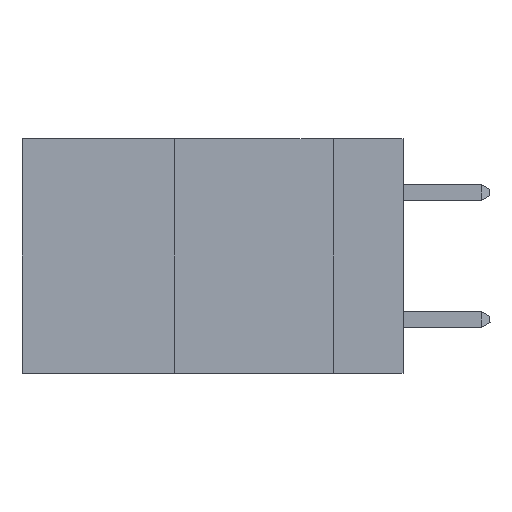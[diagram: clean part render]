
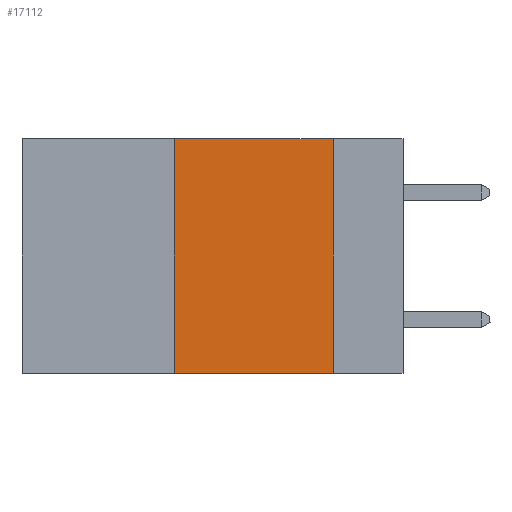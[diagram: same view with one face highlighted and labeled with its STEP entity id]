
A CAD part, left-side view. The second image highlights one B-rep face of the part: STEP entity #17112.
In plain terms, the highlighted planar face has unit normal (-1, 0, 0).
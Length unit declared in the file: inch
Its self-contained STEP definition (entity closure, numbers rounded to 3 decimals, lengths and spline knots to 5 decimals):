
#1126 = VERTEX_POINT ( 'NONE', #2800 ) ;
#1884 = CARTESIAN_POINT ( 'NONE',  ( 0., 0.11, -0.37 ) ) ;
#2019 = EDGE_CURVE ( 'NONE', #4057, #1126, #20862, .T. ) ;
#2583 = PLANE ( 'NONE',  #6562 ) ;
#2800 = CARTESIAN_POINT ( 'NONE',  ( 0., 0.36, 0. ) ) ;
#3317 = CARTESIAN_POINT ( 'NONE',  ( 0., 0.11, 0. ) ) ;
#3446 = EDGE_CURVE ( 'NONE', #4057, #5970, #21675, .T. ) ;
#4057 = VERTEX_POINT ( 'NONE', #12429 ) ;
#5388 = CARTESIAN_POINT ( 'NONE',  ( 0., 0.6, 0. ) ) ;
#5970 = VERTEX_POINT ( 'NONE', #1884 ) ;
#6185 = DIRECTION ( 'NONE',  ( 0., 0., -1. ) ) ;
#6562 = AXIS2_PLACEMENT_3D ( 'NONE', #5388, #20979, #11325 ) ;
#6912 = VERTEX_POINT ( 'NONE', #3317 ) ;
#6990 = VECTOR ( 'NONE', #25019, 39.37008 ) ;
#7381 = ORIENTED_EDGE ( 'NONE', *, *, #16291, .F. ) ;
#7469 = ORIENTED_EDGE ( 'NONE', *, *, #2019, .F. ) ;
#7756 = ORIENTED_EDGE ( 'NONE', *, *, #3446, .T. ) ;
#8862 = VECTOR ( 'NONE', #11397, 39.37008 ) ;
#9493 = DIRECTION ( 'NONE',  ( 0., 0., 1. ) ) ;
#11325 = DIRECTION ( 'NONE',  ( 0., 0., -1. ) ) ;
#11397 = DIRECTION ( 'NONE',  ( 0., -1., 0. ) ) ;
#11401 = ORIENTED_EDGE ( 'NONE', *, *, #12541, .F. ) ;
#12429 = CARTESIAN_POINT ( 'NONE',  ( 0., 0.36, -0.37 ) ) ;
#12541 = EDGE_CURVE ( 'NONE', #6912, #5970, #24641, .T. ) ;
#14245 = VECTOR ( 'NONE', #6185, 39.37008 ) ;
#15683 = VECTOR ( 'NONE', #9493, 39.37008 ) ;
#15823 = CARTESIAN_POINT ( 'NONE',  ( 0., 0.11, 0. ) ) ;
#16291 = EDGE_CURVE ( 'NONE', #1126, #6912, #22285, .T. ) ;
#17112 = ADVANCED_FACE ( 'NONE', ( #20389 ), #2583, .F. ) ;
#17359 = CARTESIAN_POINT ( 'NONE',  ( 0., 0.36, 0. ) ) ;
#17801 = EDGE_LOOP ( 'NONE', ( #11401, #7381, #7469, #7756 ) ) ;
#17897 = CARTESIAN_POINT ( 'NONE',  ( 0., 0.6, -0.37 ) ) ;
#20389 = FACE_OUTER_BOUND ( 'NONE', #17801, .T. ) ;
#20862 = LINE ( 'NONE', #17359, #15683 ) ;
#20979 = DIRECTION ( 'NONE',  ( 1., 0., 0. ) ) ;
#21247 = CARTESIAN_POINT ( 'NONE',  ( 0., 0.6, 0. ) ) ;
#21675 = LINE ( 'NONE', #17897, #8862 ) ;
#22285 = LINE ( 'NONE', #21247, #6990 ) ;
#24641 = LINE ( 'NONE', #15823, #14245 ) ;
#25019 = DIRECTION ( 'NONE',  ( 0., -1., 0. ) ) ;
